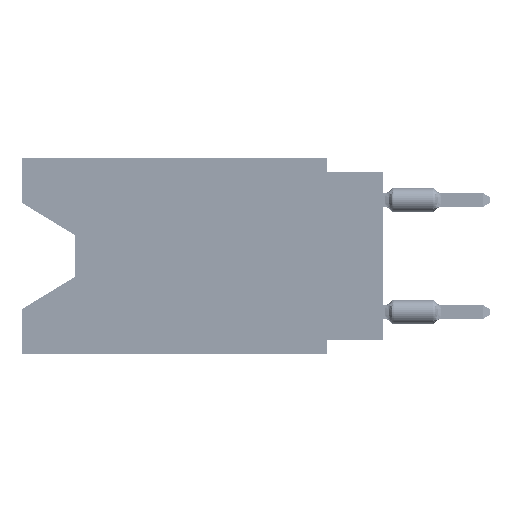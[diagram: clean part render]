
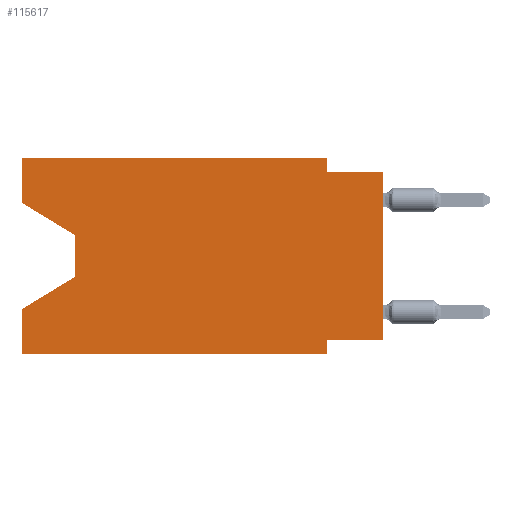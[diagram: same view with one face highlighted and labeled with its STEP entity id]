
A CAD part, left-side view. The second image highlights one B-rep face of the part: STEP entity #115617.
In plain terms, the highlighted planar face has unit normal (-1, 0, 0).
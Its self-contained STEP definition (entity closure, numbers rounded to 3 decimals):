
#791 = CARTESIAN_POINT ( 'NONE',  ( 0., 0., 0. ) ) ;
#849 = ORIENTED_EDGE ( 'NONE', *, *, #42921, .F. ) ;
#1864 = DIRECTION ( 'NONE',  ( 1., 0., 0. ) ) ;
#3373 = EDGE_CURVE ( 'NONE', #53223, #9026, #92463, .T. ) ;
#4753 = CARTESIAN_POINT ( 'NONE',  ( 0., 0., -0.635 ) ) ;
#4827 = VECTOR ( 'NONE', #106242, 1000. ) ;
#5299 = EDGE_CURVE ( 'NONE', #78418, #58433, #39350, .T. ) ;
#5456 = ORIENTED_EDGE ( 'NONE', *, *, #64181, .F. ) ;
#7790 = DIRECTION ( 'NONE',  ( 0., 0., -1. ) ) ;
#9026 = VERTEX_POINT ( 'NONE', #28286 ) ;
#9936 = ORIENTED_EDGE ( 'NONE', *, *, #26259, .T. ) ;
#15447 = CARTESIAN_POINT ( 'NONE',  ( 0., 2.54, 0. ) ) ;
#15708 = ORIENTED_EDGE ( 'NONE', *, *, #67773, .F. ) ;
#16282 = CARTESIAN_POINT ( 'NONE',  ( 0., 16.383, -2.038 ) ) ;
#20329 = CARTESIAN_POINT ( 'NONE',  ( 0., 0., -0.635 ) ) ;
#21132 = VECTOR ( 'NONE', #90152, 1000. ) ;
#21258 = VERTEX_POINT ( 'NONE', #117876 ) ;
#22355 = DIRECTION ( 'NONE',  ( 0., 0., -1. ) ) ;
#25136 = LINE ( 'NONE', #52506, #95208 ) ;
#26259 = EDGE_CURVE ( 'NONE', #87047, #58433, #93623, .T. ) ;
#26449 = VECTOR ( 'NONE', #7790, 1000. ) ;
#27309 = ORIENTED_EDGE ( 'NONE', *, *, #111386, .T. ) ;
#28286 = CARTESIAN_POINT ( 'NONE',  ( 0., 2.54, -8.255 ) ) ;
#28634 = DIRECTION ( 'NONE',  ( 0., 0., -1. ) ) ;
#28843 = DIRECTION ( 'NONE',  ( 0., -1., 0. ) ) ;
#29817 = ORIENTED_EDGE ( 'NONE', *, *, #54264, .F. ) ;
#29849 = PLANE ( 'NONE',  #93786 ) ;
#31303 = VECTOR ( 'NONE', #37879, 1000. ) ;
#31486 = CARTESIAN_POINT ( 'NONE',  ( 0., 2.54, -8.89 ) ) ;
#32410 = CARTESIAN_POINT ( 'NONE',  ( 0., 13.97, -3.505 ) ) ;
#33366 = VECTOR ( 'NONE', #113545, 1000. ) ;
#33845 = VERTEX_POINT ( 'NONE', #32410 ) ;
#34447 = CARTESIAN_POINT ( 'NONE',  ( 0., 2.54, 0. ) ) ;
#34950 = ORIENTED_EDGE ( 'NONE', *, *, #102064, .F. ) ;
#36145 = VECTOR ( 'NONE', #28843, 1000. ) ;
#37610 = VECTOR ( 'NONE', #22355, 1000. ) ;
#37879 = DIRECTION ( 'NONE',  ( 0., 0., 1. ) ) ;
#39350 = LINE ( 'NONE', #76464, #33366 ) ;
#39814 = CARTESIAN_POINT ( 'NONE',  ( 0., 13.97, -5.385 ) ) ;
#41123 = EDGE_CURVE ( 'NONE', #63950, #33845, #110524, .T. ) ;
#42921 = EDGE_CURVE ( 'NONE', #81678, #21258, #61225, .T. ) ;
#46204 = CARTESIAN_POINT ( 'NONE',  ( 0., 0., -8.255 ) ) ;
#46762 = CARTESIAN_POINT ( 'NONE',  ( 0., 13.97, -5.385 ) ) ;
#48544 = LINE ( 'NONE', #76520, #98941 ) ;
#49150 = ORIENTED_EDGE ( 'NONE', *, *, #75626, .T. ) ;
#49292 = VECTOR ( 'NONE', #80776, 1000. ) ;
#50742 = EDGE_LOOP ( 'NONE', ( #53885, #49150, #9936, #96713, #27309, #5456, #87283, #97278, #29817, #849, #15708, #34950 ) ) ;
#52506 = CARTESIAN_POINT ( 'NONE',  ( 0., 16.383, 0. ) ) ;
#53223 = VERTEX_POINT ( 'NONE', #88352 ) ;
#53885 = ORIENTED_EDGE ( 'NONE', *, *, #41123, .T. ) ;
#54264 = EDGE_CURVE ( 'NONE', #21258, #105513, #85403, .T. ) ;
#58433 = VERTEX_POINT ( 'NONE', #90372 ) ;
#59957 = VECTOR ( 'NONE', #82670, 1000. ) ;
#61225 = LINE ( 'NONE', #34447, #4827 ) ;
#62699 = CARTESIAN_POINT ( 'NONE',  ( 0., 16.383, 0. ) ) ;
#63127 = LINE ( 'NONE', #119079, #26449 ) ;
#63950 = VERTEX_POINT ( 'NONE', #118504 ) ;
#64181 = EDGE_CURVE ( 'NONE', #9026, #73880, #95985, .T. ) ;
#65186 = CARTESIAN_POINT ( 'NONE',  ( 0., 16.383, -8.89 ) ) ;
#67773 = EDGE_CURVE ( 'NONE', #97861, #81678, #48544, .T. ) ;
#72380 = DIRECTION ( 'NONE',  ( 0., 1., 0. ) ) ;
#73788 = LINE ( 'NONE', #791, #31303 ) ;
#73880 = VERTEX_POINT ( 'NONE', #31486 ) ;
#75626 = EDGE_CURVE ( 'NONE', #33845, #87047, #63127, .T. ) ;
#76464 = CARTESIAN_POINT ( 'NONE',  ( 0., 16.383, 0. ) ) ;
#76520 = CARTESIAN_POINT ( 'NONE',  ( 0., 16.383, 0. ) ) ;
#78418 = VERTEX_POINT ( 'NONE', #80788 ) ;
#80639 = EDGE_CURVE ( 'NONE', #53223, #105513, #73788, .T. ) ;
#80776 = DIRECTION ( 'NONE',  ( 0., -0.855, -0.519 ) ) ;
#80788 = CARTESIAN_POINT ( 'NONE',  ( 0., 16.383, -8.89 ) ) ;
#81678 = VERTEX_POINT ( 'NONE', #15447 ) ;
#82670 = DIRECTION ( 'NONE',  ( 0., 0.855, -0.519 ) ) ;
#85403 = LINE ( 'NONE', #20329, #36145 ) ;
#85664 = DIRECTION ( 'NONE',  ( 0., -1., 0. ) ) ;
#87047 = VERTEX_POINT ( 'NONE', #39814 ) ;
#87283 = ORIENTED_EDGE ( 'NONE', *, *, #3373, .F. ) ;
#88352 = CARTESIAN_POINT ( 'NONE',  ( 0., 0., -8.255 ) ) ;
#90152 = DIRECTION ( 'NONE',  ( 0., -1., 0. ) ) ;
#90372 = CARTESIAN_POINT ( 'NONE',  ( 0., 16.383, -6.852 ) ) ;
#92463 = LINE ( 'NONE', #46204, #102823 ) ;
#93623 = LINE ( 'NONE', #46762, #59957 ) ;
#93786 = AXIS2_PLACEMENT_3D ( 'NONE', #112549, #1864, #28634 ) ;
#95208 = VECTOR ( 'NONE', #107861, 1000. ) ;
#95985 = LINE ( 'NONE', #105080, #37610 ) ;
#96713 = ORIENTED_EDGE ( 'NONE', *, *, #5299, .F. ) ;
#97278 = ORIENTED_EDGE ( 'NONE', *, *, #80639, .T. ) ;
#97861 = VERTEX_POINT ( 'NONE', #62699 ) ;
#98941 = VECTOR ( 'NONE', #85664, 1000. ) ;
#102064 = EDGE_CURVE ( 'NONE', #63950, #97861, #25136, .T. ) ;
#102823 = VECTOR ( 'NONE', #72380, 1000. ) ;
#103452 = FACE_OUTER_BOUND ( 'NONE', #50742, .T. ) ;
#105080 = CARTESIAN_POINT ( 'NONE',  ( 0., 2.54, -8.89 ) ) ;
#105513 = VERTEX_POINT ( 'NONE', #4753 ) ;
#106242 = DIRECTION ( 'NONE',  ( 0., 0., -1. ) ) ;
#107861 = DIRECTION ( 'NONE',  ( 0., 0., 1. ) ) ;
#110524 = LINE ( 'NONE', #16282, #49292 ) ;
#111386 = EDGE_CURVE ( 'NONE', #78418, #73880, #119897, .T. ) ;
#112549 = CARTESIAN_POINT ( 'NONE',  ( 0., 16.383, 0. ) ) ;
#113545 = DIRECTION ( 'NONE',  ( 0., 0., 1. ) ) ;
#115617 = ADVANCED_FACE ( 'NONE', ( #103452 ), #29849, .F. ) ;
#117876 = CARTESIAN_POINT ( 'NONE',  ( 0., 2.54, -0.635 ) ) ;
#118504 = CARTESIAN_POINT ( 'NONE',  ( 0., 16.383, -2.038 ) ) ;
#119079 = CARTESIAN_POINT ( 'NONE',  ( 0., 13.97, -3.505 ) ) ;
#119897 = LINE ( 'NONE', #65186, #21132 ) ;
